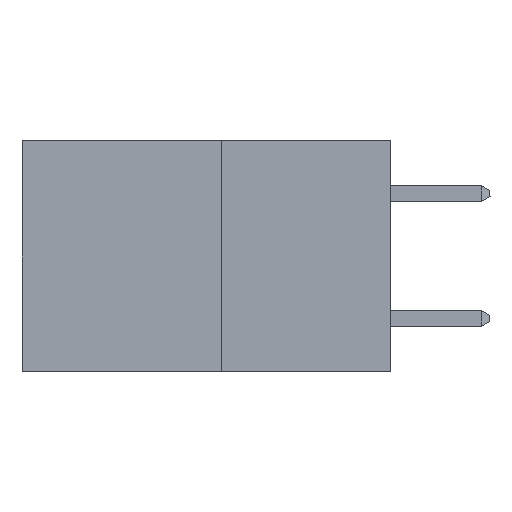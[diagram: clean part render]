
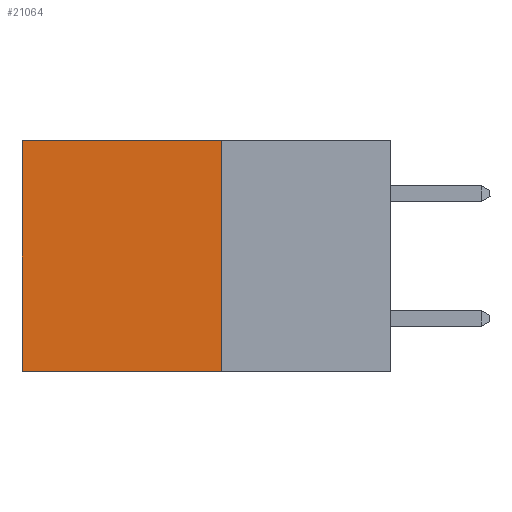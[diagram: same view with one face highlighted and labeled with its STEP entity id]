
A CAD part, left-side view. The second image highlights one B-rep face of the part: STEP entity #21064.
In plain terms, the highlighted planar face has unit normal (-1, 0, 0).
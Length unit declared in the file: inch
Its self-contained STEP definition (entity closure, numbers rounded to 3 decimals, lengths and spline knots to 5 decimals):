
#1169 = CARTESIAN_POINT ( 'NONE',  ( 0.277, 0.27, 0. ) ) ;
#1383 = EDGE_LOOP ( 'NONE', ( #13261, #24899, #15979, #21729 ) ) ;
#2181 = VERTEX_POINT ( 'NONE', #16176 ) ;
#2828 = LINE ( 'NONE', #4463, #13232 ) ;
#2952 = LINE ( 'NONE', #28465, #26501 ) ;
#4463 = CARTESIAN_POINT ( 'NONE',  ( 0.277, 0.27, -0.37 ) ) ;
#4556 = DIRECTION ( 'NONE',  ( 0., 1., 0. ) ) ;
#5068 = VERTEX_POINT ( 'NONE', #9319 ) ;
#6469 = CARTESIAN_POINT ( 'NONE',  ( 0.277, 0.27, -0.37 ) ) ;
#6652 = EDGE_CURVE ( 'NONE', #12037, #5068, #10969, .T. ) ;
#6925 = PLANE ( 'NONE',  #14002 ) ;
#9109 = CARTESIAN_POINT ( 'NONE',  ( 0.277, 0.27, -0.37 ) ) ;
#9209 = DIRECTION ( 'NONE',  ( 0., 0., -1. ) ) ;
#9319 = CARTESIAN_POINT ( 'NONE',  ( 0.277, 0.59, 0. ) ) ;
#10935 = LINE ( 'NONE', #6469, #23369 ) ;
#10969 = LINE ( 'NONE', #1169, #27906 ) ;
#12037 = VERTEX_POINT ( 'NONE', #21822 ) ;
#13232 = VECTOR ( 'NONE', #4556, 39.37008 ) ;
#13261 = ORIENTED_EDGE ( 'NONE', *, *, #14432, .T. ) ;
#14002 = AXIS2_PLACEMENT_3D ( 'NONE', #9109, #22402, #9209 ) ;
#14432 = EDGE_CURVE ( 'NONE', #5068, #2181, #2952, .T. ) ;
#15222 = DIRECTION ( 'NONE',  ( 0., 0., -1. ) ) ;
#15979 = ORIENTED_EDGE ( 'NONE', *, *, #22331, .F. ) ;
#16176 = CARTESIAN_POINT ( 'NONE',  ( 0.277, 0.59, -0.37 ) ) ;
#16742 = DIRECTION ( 'NONE',  ( 0., 1., 0. ) ) ;
#16743 = VERTEX_POINT ( 'NONE', #24984 ) ;
#19991 = EDGE_CURVE ( 'NONE', #16743, #2181, #2828, .T. ) ;
#21064 = ADVANCED_FACE ( 'NONE', ( #25972 ), #6925, .F. ) ;
#21729 = ORIENTED_EDGE ( 'NONE', *, *, #6652, .T. ) ;
#21822 = CARTESIAN_POINT ( 'NONE',  ( 0.277, 0.27, 0. ) ) ;
#21932 = DIRECTION ( 'NONE',  ( 0., 0., -1. ) ) ;
#22331 = EDGE_CURVE ( 'NONE', #12037, #16743, #10935, .T. ) ;
#22402 = DIRECTION ( 'NONE',  ( 1., 0., 0. ) ) ;
#23369 = VECTOR ( 'NONE', #21932, 39.37008 ) ;
#24899 = ORIENTED_EDGE ( 'NONE', *, *, #19991, .F. ) ;
#24984 = CARTESIAN_POINT ( 'NONE',  ( 0.277, 0.27, -0.37 ) ) ;
#25972 = FACE_OUTER_BOUND ( 'NONE', #1383, .T. ) ;
#26501 = VECTOR ( 'NONE', #15222, 39.37008 ) ;
#27906 = VECTOR ( 'NONE', #16742, 39.37008 ) ;
#28465 = CARTESIAN_POINT ( 'NONE',  ( 0.277, 0.59, -0.37 ) ) ;
